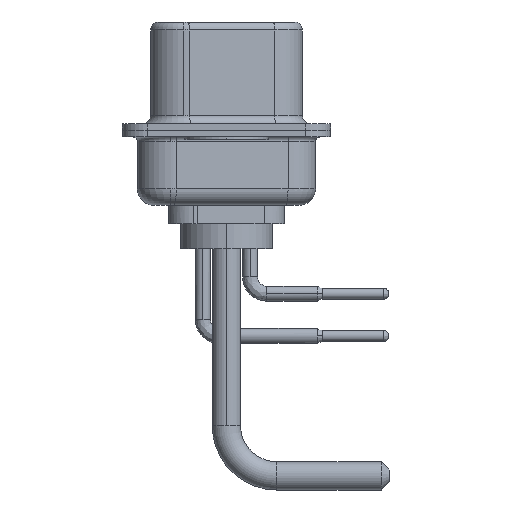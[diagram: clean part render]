
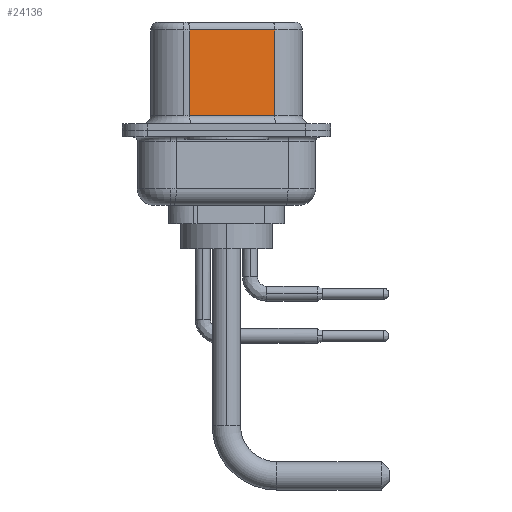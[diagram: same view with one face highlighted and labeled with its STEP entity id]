
A CAD part, left-side view. The second image highlights one B-rep face of the part: STEP entity #24136.
In plain terms, the highlighted planar face has unit normal (-0.985, -0.174, 0).
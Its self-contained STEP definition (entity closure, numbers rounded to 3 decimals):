
#341 = CARTESIAN_POINT ( 'NONE',  ( 4.58, -2.897, 6.52 ) ) ;
#750 = VERTEX_POINT ( 'NONE', #14363 ) ;
#855 = EDGE_CURVE ( 'NONE', #3943, #16522, #19097, .T. ) ;
#1853 = LINE ( 'NONE', #26465, #16238 ) ;
#3750 = DIRECTION ( 'NONE',  ( -0.174, 0.985, 0. ) ) ;
#3931 = LINE ( 'NONE', #7703, #9538 ) ;
#3943 = VERTEX_POINT ( 'NONE', #20697 ) ;
#5531 = AXIS2_PLACEMENT_3D ( 'NONE', #341, #21405, #21014 ) ;
#6193 = ORIENTED_EDGE ( 'NONE', *, *, #855, .T. ) ;
#6198 = CARTESIAN_POINT ( 'NONE',  ( 4.58, -2.897, 6.02 ) ) ;
#7445 = CARTESIAN_POINT ( 'NONE',  ( 4.58, -2.897, 0.9 ) ) ;
#7703 = CARTESIAN_POINT ( 'NONE',  ( 4.58, -2.897, 6.52 ) ) ;
#8714 = FACE_OUTER_BOUND ( 'NONE', #19154, .T. ) ;
#9538 = VECTOR ( 'NONE', #12177, 1000. ) ;
#11849 = ORIENTED_EDGE ( 'NONE', *, *, #24828, .F. ) ;
#12177 = DIRECTION ( 'NONE',  ( 0., 0., -1. ) ) ;
#13160 = PLANE ( 'NONE',  #5531 ) ;
#13422 = VECTOR ( 'NONE', #23688, 1000. ) ;
#14363 = CARTESIAN_POINT ( 'NONE',  ( 3.68, 2.203, 6.02 ) ) ;
#15435 = CARTESIAN_POINT ( 'NONE',  ( 4.58, -2.897, 0.9 ) ) ;
#16238 = VECTOR ( 'NONE', #3750, 1000. ) ;
#16356 = ORIENTED_EDGE ( 'NONE', *, *, #22235, .T. ) ;
#16522 = VERTEX_POINT ( 'NONE', #7445 ) ;
#18673 = LINE ( 'NONE', #22727, #24353 ) ;
#19012 = EDGE_CURVE ( 'NONE', #750, #3943, #18673, .T. ) ;
#19097 = LINE ( 'NONE', #15435, #13422 ) ;
#19154 = EDGE_LOOP ( 'NONE', ( #11849, #16356, #20966, #6193 ) ) ;
#19381 = VERTEX_POINT ( 'NONE', #6198 ) ;
#20697 = CARTESIAN_POINT ( 'NONE',  ( 3.68, 2.203, 0.9 ) ) ;
#20703 = DIRECTION ( 'NONE',  ( 0., 0., -1. ) ) ;
#20966 = ORIENTED_EDGE ( 'NONE', *, *, #19012, .T. ) ;
#21014 = DIRECTION ( 'NONE',  ( -0.174, 0.985, 0. ) ) ;
#21405 = DIRECTION ( 'NONE',  ( 0.985, 0.174, 0. ) ) ;
#22235 = EDGE_CURVE ( 'NONE', #19381, #750, #1853, .T. ) ;
#22727 = CARTESIAN_POINT ( 'NONE',  ( 3.68, 2.203, 6.52 ) ) ;
#23688 = DIRECTION ( 'NONE',  ( 0.174, -0.985, 0. ) ) ;
#24136 = ADVANCED_FACE ( 'NONE', ( #8714 ), #13160, .F. ) ;
#24353 = VECTOR ( 'NONE', #20703, 1000. ) ;
#24828 = EDGE_CURVE ( 'NONE', #19381, #16522, #3931, .T. ) ;
#26465 = CARTESIAN_POINT ( 'NONE',  ( 4.58, -2.897, 6.02 ) ) ;
